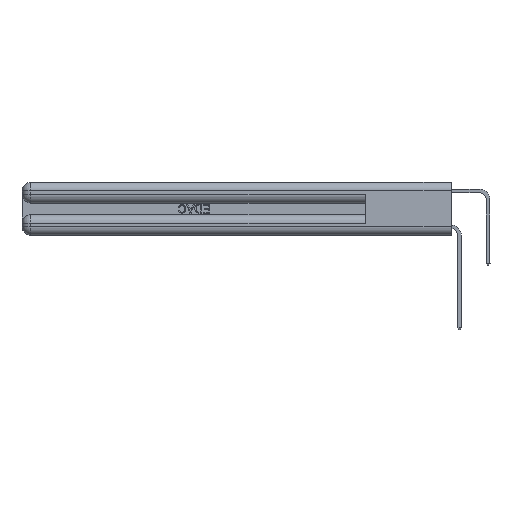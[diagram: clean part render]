
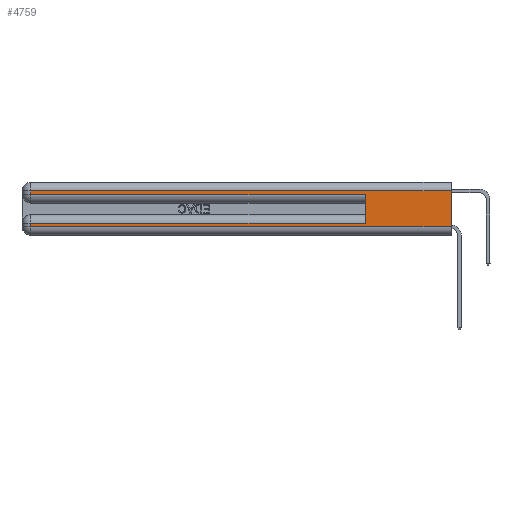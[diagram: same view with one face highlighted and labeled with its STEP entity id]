
A CAD part, left-side view. The second image highlights one B-rep face of the part: STEP entity #4759.
In plain terms, the highlighted planar face has unit normal (-1, 0, 0).
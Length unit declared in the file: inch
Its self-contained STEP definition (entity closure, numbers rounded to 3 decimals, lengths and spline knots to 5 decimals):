
#586 = CARTESIAN_POINT ( 'NONE',  ( 0., 0., 0.31 ) ) ;
#1029 = EDGE_CURVE ( 'NONE', #1923, #23285, #3183, .T. ) ;
#1923 = VERTEX_POINT ( 'NONE', #10383 ) ;
#2035 = DIRECTION ( 'NONE',  ( 1., 0., 0. ) ) ;
#2204 = FACE_OUTER_BOUND ( 'NONE', #9069, .T. ) ;
#2415 = EDGE_CURVE ( 'NONE', #2529, #29061, #27027, .T. ) ;
#2529 = VERTEX_POINT ( 'NONE', #3051 ) ;
#2533 = AXIS2_PLACEMENT_3D ( 'NONE', #31215, #2035, #7379 ) ;
#3051 = CARTESIAN_POINT ( 'NONE',  ( 0., 2.94, 0.06 ) ) ;
#3183 = LINE ( 'NONE', #586, #31224 ) ;
#3647 = CARTESIAN_POINT ( 'NONE',  ( 0., 0., 0.085 ) ) ;
#4115 = DIRECTION ( 'NONE',  ( 0., 0., 1. ) ) ;
#4282 = LINE ( 'NONE', #9297, #21984 ) ;
#4394 = EDGE_CURVE ( 'NONE', #23285, #9947, #24563, .T. ) ;
#4759 = ADVANCED_FACE ( 'NONE', ( #2204 ), #25812, .F. ) ;
#5870 = EDGE_CURVE ( 'NONE', #32880, #25452, #27443, .T. ) ;
#7379 = DIRECTION ( 'NONE',  ( 0., 0., -1. ) ) ;
#8126 = EDGE_CURVE ( 'NONE', #9947, #14300, #26773, .T. ) ;
#9069 = EDGE_LOOP ( 'NONE', ( #29920, #29801, #12225, #19007, #19781, #9488, #10468, #11859 ) ) ;
#9297 = CARTESIAN_POINT ( 'NONE',  ( 0., 0., 0.37 ) ) ;
#9488 = ORIENTED_EDGE ( 'NONE', *, *, #5870, .T. ) ;
#9694 = CARTESIAN_POINT ( 'NONE',  ( 0., 0., 0.06 ) ) ;
#9947 = VERTEX_POINT ( 'NONE', #21350 ) ;
#10383 = CARTESIAN_POINT ( 'NONE',  ( 0., 0., 0.31 ) ) ;
#10468 = ORIENTED_EDGE ( 'NONE', *, *, #30798, .T. ) ;
#10735 = CARTESIAN_POINT ( 'NONE',  ( 0., 2.94, 0.37 ) ) ;
#11340 = DIRECTION ( 'NONE',  ( 0., 0., -1. ) ) ;
#11859 = ORIENTED_EDGE ( 'NONE', *, *, #2415, .T. ) ;
#12225 = ORIENTED_EDGE ( 'NONE', *, *, #4394, .T. ) ;
#12228 = VECTOR ( 'NONE', #14166, 39.37008 ) ;
#13651 = CARTESIAN_POINT ( 'NONE',  ( 0., 0., 0.06 ) ) ;
#14131 = CARTESIAN_POINT ( 'NONE',  ( 0., 2.94, 0.37 ) ) ;
#14166 = DIRECTION ( 'NONE',  ( 0., -1., 0. ) ) ;
#14241 = DIRECTION ( 'NONE',  ( 0., 1., 0. ) ) ;
#14300 = VERTEX_POINT ( 'NONE', #27691 ) ;
#15261 = EDGE_CURVE ( 'NONE', #1923, #29061, #4282, .T. ) ;
#16441 = VECTOR ( 'NONE', #14241, 39.37008 ) ;
#17483 = CARTESIAN_POINT ( 'NONE',  ( 0., 0.6, 0.145 ) ) ;
#18906 = LINE ( 'NONE', #10735, #19914 ) ;
#19007 = ORIENTED_EDGE ( 'NONE', *, *, #8126, .T. ) ;
#19781 = ORIENTED_EDGE ( 'NONE', *, *, #28290, .F. ) ;
#19904 = DIRECTION ( 'NONE',  ( 0., 0., -1. ) ) ;
#19912 = LINE ( 'NONE', #17483, #34262 ) ;
#19914 = VECTOR ( 'NONE', #31960, 39.37008 ) ;
#21350 = CARTESIAN_POINT ( 'NONE',  ( 0., 2.94, 0.285 ) ) ;
#21984 = VECTOR ( 'NONE', #19904, 39.37008 ) ;
#22488 = VECTOR ( 'NONE', #11340, 39.37008 ) ;
#22837 = CARTESIAN_POINT ( 'NONE',  ( 0., 2.94, 0.31 ) ) ;
#23246 = CARTESIAN_POINT ( 'NONE',  ( 0., 2.94, 0.085 ) ) ;
#23285 = VERTEX_POINT ( 'NONE', #22837 ) ;
#24563 = LINE ( 'NONE', #14131, #22488 ) ;
#25452 = VERTEX_POINT ( 'NONE', #23246 ) ;
#25792 = DIRECTION ( 'NONE',  ( 0., -1., 0. ) ) ;
#25812 = PLANE ( 'NONE',  #2533 ) ;
#26773 = LINE ( 'NONE', #34276, #33223 ) ;
#27027 = LINE ( 'NONE', #13651, #12228 ) ;
#27443 = LINE ( 'NONE', #3647, #16441 ) ;
#27691 = CARTESIAN_POINT ( 'NONE',  ( 0., 0.6, 0.285 ) ) ;
#28290 = EDGE_CURVE ( 'NONE', #32880, #14300, #19912, .T. ) ;
#29061 = VERTEX_POINT ( 'NONE', #9694 ) ;
#29801 = ORIENTED_EDGE ( 'NONE', *, *, #1029, .T. ) ;
#29920 = ORIENTED_EDGE ( 'NONE', *, *, #15261, .F. ) ;
#30798 = EDGE_CURVE ( 'NONE', #25452, #2529, #18906, .T. ) ;
#31215 = CARTESIAN_POINT ( 'NONE',  ( 0., 0., 0.37 ) ) ;
#31224 = VECTOR ( 'NONE', #32379, 39.37008 ) ;
#31960 = DIRECTION ( 'NONE',  ( 0., 0., -1. ) ) ;
#32379 = DIRECTION ( 'NONE',  ( 0., 1., 0. ) ) ;
#32880 = VERTEX_POINT ( 'NONE', #33264 ) ;
#33223 = VECTOR ( 'NONE', #25792, 39.37008 ) ;
#33264 = CARTESIAN_POINT ( 'NONE',  ( 0., 0.6, 0.085 ) ) ;
#34262 = VECTOR ( 'NONE', #4115, 39.37008 ) ;
#34276 = CARTESIAN_POINT ( 'NONE',  ( 0., 0., 0.285 ) ) ;
